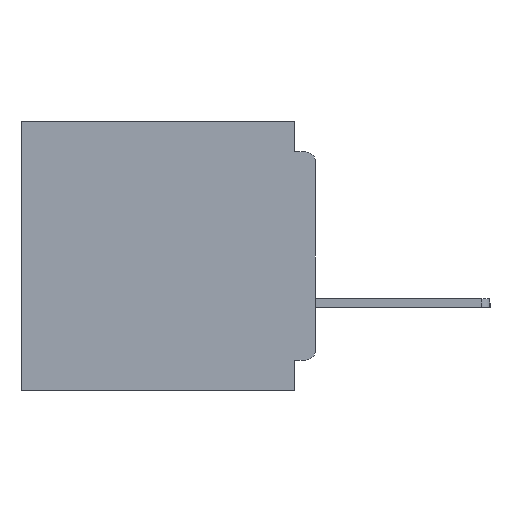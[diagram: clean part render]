
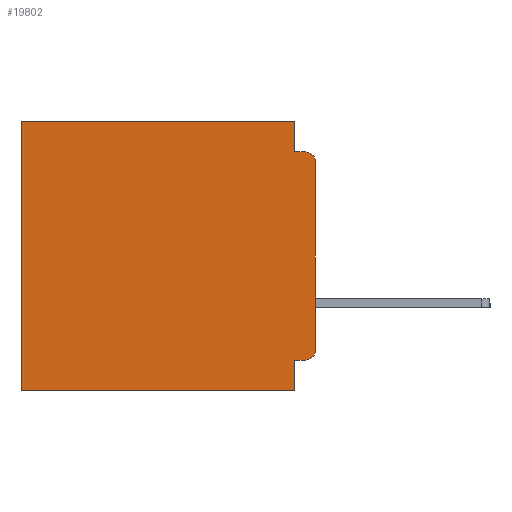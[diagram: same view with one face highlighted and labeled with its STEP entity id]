
A CAD part, left-side view. The second image highlights one B-rep face of the part: STEP entity #19802.
In plain terms, the highlighted planar face has unit normal (-1, 0, 0).
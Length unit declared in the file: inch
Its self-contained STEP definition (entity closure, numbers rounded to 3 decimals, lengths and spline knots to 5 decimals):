
#449 = CARTESIAN_POINT ( 'NONE',  ( 0.3, 0., -0.4 ) ) ;
#713 = VERTEX_POINT ( 'NONE', #15649 ) ;
#904 = AXIS2_PLACEMENT_3D ( 'NONE', #34029, #18079, #2071 ) ;
#972 = EDGE_CURVE ( 'NONE', #7812, #8951, #6363, .T. ) ;
#1433 = VECTOR ( 'NONE', #12953, 39.37008 ) ;
#1679 = EDGE_CURVE ( 'NONE', #9302, #11971, #5044, .T. ) ;
#1818 = DIRECTION ( 'NONE',  ( 0., 0., -1. ) ) ;
#2071 = DIRECTION ( 'NONE',  ( 0., 0., -1. ) ) ;
#2242 = LINE ( 'NONE', #23582, #1433 ) ;
#2831 = AXIS2_PLACEMENT_3D ( 'NONE', #20680, #4718, #23396 ) ;
#3651 = LINE ( 'NONE', #17764, #16990 ) ;
#3653 = VERTEX_POINT ( 'NONE', #15668 ) ;
#4487 = DIRECTION ( 'NONE',  ( 0., -1., 0. ) ) ;
#4718 = DIRECTION ( 'NONE',  ( -1., 0., 0. ) ) ;
#4846 = FACE_OUTER_BOUND ( 'NONE', #23803, .T. ) ;
#4886 = VECTOR ( 'NONE', #18658, 39.37008 ) ;
#5044 = LINE ( 'NONE', #34298, #25528 ) ;
#5051 = CARTESIAN_POINT ( 'NONE',  ( 0.3, 0.031, -0.4 ) ) ;
#5144 = CARTESIAN_POINT ( 'NONE',  ( 0.3, 0.437, 0. ) ) ;
#5661 = ORIENTED_EDGE ( 'NONE', *, *, #16900, .T. ) ;
#6363 = LINE ( 'NONE', #16335, #33874 ) ;
#6857 = EDGE_CURVE ( 'NONE', #7812, #18744, #9216, .T. ) ;
#7198 = AXIS2_PLACEMENT_3D ( 'NONE', #15117, #17806, #1818 ) ;
#7679 = ORIENTED_EDGE ( 'NONE', *, *, #27473, .F. ) ;
#7812 = VERTEX_POINT ( 'NONE', #26825 ) ;
#8951 = VERTEX_POINT ( 'NONE', #26276 ) ;
#9216 = LINE ( 'NONE', #25772, #21703 ) ;
#9302 = VERTEX_POINT ( 'NONE', #14436 ) ;
#9648 = VERTEX_POINT ( 'NONE', #34554 ) ;
#10331 = VECTOR ( 'NONE', #24630, 39.37008 ) ;
#11172 = CIRCLE ( 'NONE', #2831, 0.015 ) ;
#11753 = CARTESIAN_POINT ( 'NONE',  ( 0.3, 0., -0.34 ) ) ;
#11971 = VERTEX_POINT ( 'NONE', #5051 ) ;
#12482 = PLANE ( 'NONE',  #7198 ) ;
#12953 = DIRECTION ( 'NONE',  ( 0., 0., -1. ) ) ;
#13047 = DIRECTION ( 'NONE',  ( 0., 0., -1. ) ) ;
#13125 = ORIENTED_EDGE ( 'NONE', *, *, #972, .F. ) ;
#13418 = VECTOR ( 'NONE', #15381, 39.37008 ) ;
#14436 = CARTESIAN_POINT ( 'NONE',  ( 0.3, 0.031, -0.355 ) ) ;
#15117 = CARTESIAN_POINT ( 'NONE',  ( 0.3, 0., -0.4 ) ) ;
#15381 = DIRECTION ( 'NONE',  ( 0., 0., -1. ) ) ;
#15649 = CARTESIAN_POINT ( 'NONE',  ( 0.3, 0.015, -0.045 ) ) ;
#15668 = CARTESIAN_POINT ( 'NONE',  ( 0.3, 0.015, -0.355 ) ) ;
#16218 = EDGE_CURVE ( 'NONE', #8951, #713, #3651, .T. ) ;
#16335 = CARTESIAN_POINT ( 'NONE',  ( 0.3, 0.031, 0. ) ) ;
#16900 = EDGE_CURVE ( 'NONE', #18744, #24241, #33846, .T. ) ;
#16990 = VECTOR ( 'NONE', #4487, 39.37008 ) ;
#17409 = LINE ( 'NONE', #449, #10331 ) ;
#17764 = CARTESIAN_POINT ( 'NONE',  ( 0.3, 0., -0.045 ) ) ;
#17806 = DIRECTION ( 'NONE',  ( 1., 0., 0. ) ) ;
#18079 = DIRECTION ( 'NONE',  ( -1., 0., 0. ) ) ;
#18573 = ORIENTED_EDGE ( 'NONE', *, *, #32613, .T. ) ;
#18653 = EDGE_CURVE ( 'NONE', #9648, #713, #26669, .T. ) ;
#18658 = DIRECTION ( 'NONE',  ( 0., 1., 0. ) ) ;
#18744 = VERTEX_POINT ( 'NONE', #5144 ) ;
#18956 = EDGE_CURVE ( 'NONE', #11971, #24241, #17409, .T. ) ;
#19387 = EDGE_CURVE ( 'NONE', #3653, #9302, #25355, .T. ) ;
#19635 = DIRECTION ( 'NONE',  ( 0., 0., -1. ) ) ;
#19769 = CARTESIAN_POINT ( 'NONE',  ( 0.3, 0., -0.355 ) ) ;
#19802 = ADVANCED_FACE ( 'NONE', ( #4846 ), #12482, .F. ) ;
#20011 = CARTESIAN_POINT ( 'NONE',  ( 0.3, 0.437, -0.4 ) ) ;
#20266 = VERTEX_POINT ( 'NONE', #11753 ) ;
#20680 = CARTESIAN_POINT ( 'NONE',  ( 0.3, 0.015, -0.34 ) ) ;
#21703 = VECTOR ( 'NONE', #25845, 39.37008 ) ;
#23143 = ORIENTED_EDGE ( 'NONE', *, *, #18653, .T. ) ;
#23180 = ORIENTED_EDGE ( 'NONE', *, *, #1679, .F. ) ;
#23396 = DIRECTION ( 'NONE',  ( 0., 0., -1. ) ) ;
#23582 = CARTESIAN_POINT ( 'NONE',  ( 0.3, 0., -0.4 ) ) ;
#23803 = EDGE_LOOP ( 'NONE', ( #7679, #23143, #31918, #13125, #29885, #5661, #27784, #23180, #24872, #18573 ) ) ;
#24241 = VERTEX_POINT ( 'NONE', #20011 ) ;
#24630 = DIRECTION ( 'NONE',  ( 0., 1., 0. ) ) ;
#24872 = ORIENTED_EDGE ( 'NONE', *, *, #19387, .F. ) ;
#25355 = LINE ( 'NONE', #19769, #4886 ) ;
#25528 = VECTOR ( 'NONE', #13047, 39.37008 ) ;
#25772 = CARTESIAN_POINT ( 'NONE',  ( 0.3, 0., 0. ) ) ;
#25845 = DIRECTION ( 'NONE',  ( 0., 1., 0. ) ) ;
#26276 = CARTESIAN_POINT ( 'NONE',  ( 0.3, 0.031, -0.045 ) ) ;
#26669 = CIRCLE ( 'NONE', #904, 0.015 ) ;
#26825 = CARTESIAN_POINT ( 'NONE',  ( 0.3, 0.031, 0. ) ) ;
#27473 = EDGE_CURVE ( 'NONE', #9648, #20266, #2242, .T. ) ;
#27784 = ORIENTED_EDGE ( 'NONE', *, *, #18956, .F. ) ;
#29885 = ORIENTED_EDGE ( 'NONE', *, *, #6857, .T. ) ;
#31411 = CARTESIAN_POINT ( 'NONE',  ( 0.3, 0.437, -0.4 ) ) ;
#31918 = ORIENTED_EDGE ( 'NONE', *, *, #16218, .F. ) ;
#32613 = EDGE_CURVE ( 'NONE', #3653, #20266, #11172, .T. ) ;
#33846 = LINE ( 'NONE', #31411, #13418 ) ;
#33874 = VECTOR ( 'NONE', #19635, 39.37008 ) ;
#34029 = CARTESIAN_POINT ( 'NONE',  ( 0.3, 0.015, -0.06 ) ) ;
#34298 = CARTESIAN_POINT ( 'NONE',  ( 0.3, 0.031, -0.4 ) ) ;
#34554 = CARTESIAN_POINT ( 'NONE',  ( 0.3, 0., -0.06 ) ) ;
